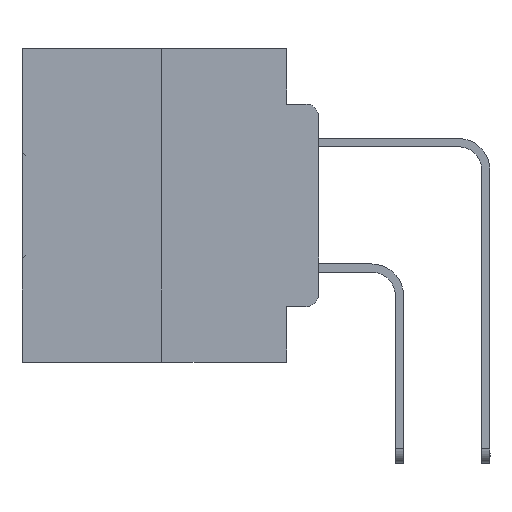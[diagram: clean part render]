
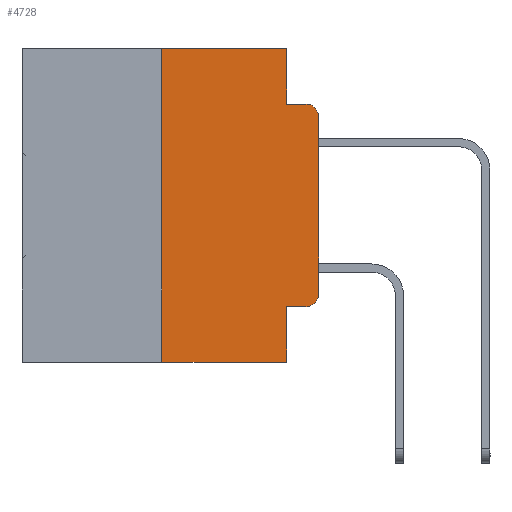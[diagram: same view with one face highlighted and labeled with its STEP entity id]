
A CAD part, left-side view. The second image highlights one B-rep face of the part: STEP entity #4728.
In plain terms, the highlighted planar face has unit normal (-1, 0, 0).
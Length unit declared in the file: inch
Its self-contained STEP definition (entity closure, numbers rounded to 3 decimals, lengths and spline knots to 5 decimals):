
#63 = VECTOR ( 'NONE', #20644, 39.37008 ) ;
#147 = ORIENTED_EDGE ( 'NONE', *, *, #33290, .T. ) ;
#407 = DIRECTION ( 'NONE',  ( 0., 0., -1. ) ) ;
#959 = VECTOR ( 'NONE', #2233, 39.37008 ) ;
#1597 = DIRECTION ( 'NONE',  ( 0., -1., 0. ) ) ;
#2233 = DIRECTION ( 'NONE',  ( 0., -1., 0. ) ) ;
#3064 = CARTESIAN_POINT ( 'NONE',  ( 0., 0.25, 0. ) ) ;
#3184 = EDGE_CURVE ( 'NONE', #17152, #15064, #17881, .T. ) ;
#3405 = VECTOR ( 'NONE', #27245, 39.37008 ) ;
#3421 = CARTESIAN_POINT ( 'NONE',  ( 0., 0., 0. ) ) ;
#4676 = DIRECTION ( 'NONE',  ( -1., 0., 0. ) ) ;
#4728 = ADVANCED_FACE ( 'NONE', ( #24835 ), #13177, .F. ) ;
#5067 = ORIENTED_EDGE ( 'NONE', *, *, #30198, .T. ) ;
#5267 = CIRCLE ( 'NONE', #17912, 0.02 ) ;
#7038 = LINE ( 'NONE', #25852, #63 ) ;
#7295 = EDGE_CURVE ( 'NONE', #24796, #30129, #31283, .T. ) ;
#7690 = EDGE_CURVE ( 'NONE', #24796, #19600, #21400, .T. ) ;
#8893 = CARTESIAN_POINT ( 'NONE',  ( 0., 0., -0.1085 ) ) ;
#9349 = CARTESIAN_POINT ( 'NONE',  ( 0., 0., -0.3915 ) ) ;
#9593 = CARTESIAN_POINT ( 'NONE',  ( 0., 0.02, -0.0885 ) ) ;
#9641 = DIRECTION ( 'NONE',  ( 0., -1., 0. ) ) ;
#9734 = CARTESIAN_POINT ( 'NONE',  ( 0., 0.02, -0.3915 ) ) ;
#9826 = DIRECTION ( 'NONE',  ( 0., 0., -1. ) ) ;
#10015 = CARTESIAN_POINT ( 'NONE',  ( 0., 0.051, -0.4115 ) ) ;
#10375 = VERTEX_POINT ( 'NONE', #3064 ) ;
#10382 = LINE ( 'NONE', #3421, #3405 ) ;
#11760 = LINE ( 'NONE', #31434, #17895 ) ;
#12428 = DIRECTION ( 'NONE',  ( -1., 0., 0. ) ) ;
#13177 = PLANE ( 'NONE',  #17754 ) ;
#13637 = VECTOR ( 'NONE', #1597, 39.37008 ) ;
#14799 = ORIENTED_EDGE ( 'NONE', *, *, #7690, .F. ) ;
#14909 = CARTESIAN_POINT ( 'NONE',  ( 0., 0.051, 0. ) ) ;
#14944 = DIRECTION ( 'NONE',  ( 0., 0., -1. ) ) ;
#15006 = CARTESIAN_POINT ( 'NONE',  ( 0., 0.051, -0.0885 ) ) ;
#15064 = VERTEX_POINT ( 'NONE', #9593 ) ;
#15146 = ORIENTED_EDGE ( 'NONE', *, *, #7295, .T. ) ;
#15692 = DIRECTION ( 'NONE',  ( 0., 0., -1. ) ) ;
#15804 = DIRECTION ( 'NONE',  ( 1., 0., 0. ) ) ;
#16260 = VECTOR ( 'NONE', #9641, 39.37008 ) ;
#17152 = VERTEX_POINT ( 'NONE', #28865 ) ;
#17343 = EDGE_CURVE ( 'NONE', #32015, #18112, #10382, .T. ) ;
#17585 = EDGE_CURVE ( 'NONE', #10375, #18879, #18518, .T. ) ;
#17588 = CARTESIAN_POINT ( 'NONE',  ( 0., 0.051, 0. ) ) ;
#17698 = VECTOR ( 'NONE', #9826, 39.37008 ) ;
#17754 = AXIS2_PLACEMENT_3D ( 'NONE', #31466, #15804, #15692 ) ;
#17881 = LINE ( 'NONE', #15006, #16260 ) ;
#17895 = VECTOR ( 'NONE', #407, 39.37008 ) ;
#17912 = AXIS2_PLACEMENT_3D ( 'NONE', #9734, #4676, #30657 ) ;
#18112 = VERTEX_POINT ( 'NONE', #8893 ) ;
#18458 = EDGE_CURVE ( 'NONE', #22525, #19600, #7038, .T. ) ;
#18496 = EDGE_CURVE ( 'NONE', #22525, #10375, #33170, .T. ) ;
#18518 = LINE ( 'NONE', #22875, #13637 ) ;
#18879 = VERTEX_POINT ( 'NONE', #14909 ) ;
#19600 = VERTEX_POINT ( 'NONE', #28720 ) ;
#19921 = CARTESIAN_POINT ( 'NONE',  ( 0., 0.25, -0.5 ) ) ;
#20013 = CARTESIAN_POINT ( 'NONE',  ( 0., 0.051, -0.4115 ) ) ;
#20376 = AXIS2_PLACEMENT_3D ( 'NONE', #25400, #12428, #14944 ) ;
#20644 = DIRECTION ( 'NONE',  ( 0., -1., 0. ) ) ;
#21400 = LINE ( 'NONE', #17588, #17698 ) ;
#22335 = CARTESIAN_POINT ( 'NONE',  ( 0., 0.02, -0.4115 ) ) ;
#22525 = VERTEX_POINT ( 'NONE', #19921 ) ;
#22875 = CARTESIAN_POINT ( 'NONE',  ( 0., 0.473, 0. ) ) ;
#23572 = ORIENTED_EDGE ( 'NONE', *, *, #17585, .F. ) ;
#24796 = VERTEX_POINT ( 'NONE', #20013 ) ;
#24835 = FACE_OUTER_BOUND ( 'NONE', #28388, .T. ) ;
#25125 = CIRCLE ( 'NONE', #20376, 0.02 ) ;
#25400 = CARTESIAN_POINT ( 'NONE',  ( 0., 0.02, -0.1085 ) ) ;
#25612 = EDGE_CURVE ( 'NONE', #18879, #17152, #11760, .T. ) ;
#25852 = CARTESIAN_POINT ( 'NONE',  ( 0., 0.473, -0.5 ) ) ;
#25956 = ORIENTED_EDGE ( 'NONE', *, *, #18458, .T. ) ;
#26956 = ORIENTED_EDGE ( 'NONE', *, *, #18496, .F. ) ;
#27018 = ORIENTED_EDGE ( 'NONE', *, *, #25612, .F. ) ;
#27245 = DIRECTION ( 'NONE',  ( 0., 0., 1. ) ) ;
#28388 = EDGE_LOOP ( 'NONE', ( #31907, #147, #33139, #27018, #23572, #26956, #25956, #14799, #15146, #5067 ) ) ;
#28720 = CARTESIAN_POINT ( 'NONE',  ( 0., 0.051, -0.5 ) ) ;
#28865 = CARTESIAN_POINT ( 'NONE',  ( 0., 0.051, -0.0885 ) ) ;
#29008 = DIRECTION ( 'NONE',  ( 0., 0., 1. ) ) ;
#30129 = VERTEX_POINT ( 'NONE', #22335 ) ;
#30198 = EDGE_CURVE ( 'NONE', #30129, #32015, #5267, .T. ) ;
#30657 = DIRECTION ( 'NONE',  ( 0., 0., -1. ) ) ;
#30725 = VECTOR ( 'NONE', #29008, 39.37008 ) ;
#31283 = LINE ( 'NONE', #10015, #959 ) ;
#31434 = CARTESIAN_POINT ( 'NONE',  ( 0., 0.051, 0. ) ) ;
#31466 = CARTESIAN_POINT ( 'NONE',  ( 0., 0.473, 0. ) ) ;
#31518 = CARTESIAN_POINT ( 'NONE',  ( 0., 0.25, 0. ) ) ;
#31907 = ORIENTED_EDGE ( 'NONE', *, *, #17343, .T. ) ;
#32015 = VERTEX_POINT ( 'NONE', #9349 ) ;
#33139 = ORIENTED_EDGE ( 'NONE', *, *, #3184, .F. ) ;
#33170 = LINE ( 'NONE', #31518, #30725 ) ;
#33290 = EDGE_CURVE ( 'NONE', #18112, #15064, #25125, .T. ) ;
